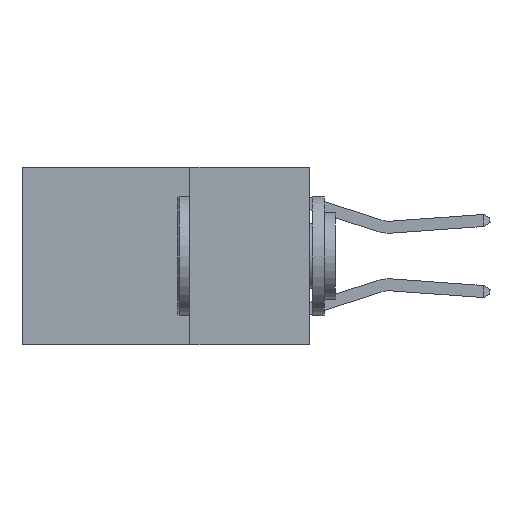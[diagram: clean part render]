
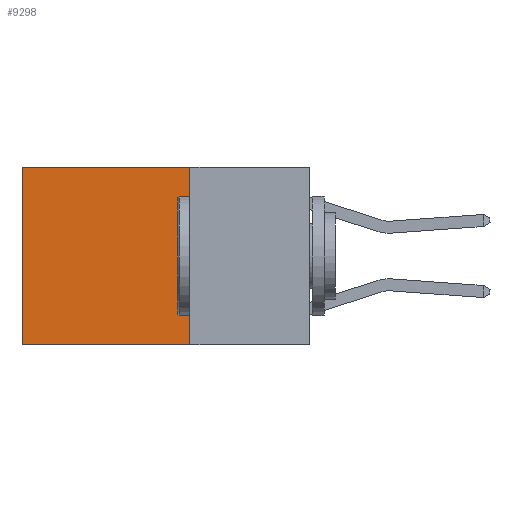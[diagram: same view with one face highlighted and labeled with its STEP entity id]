
A CAD part, left-side view. The second image highlights one B-rep face of the part: STEP entity #9298.
In plain terms, the highlighted planar face has unit normal (-1, 0, 0).
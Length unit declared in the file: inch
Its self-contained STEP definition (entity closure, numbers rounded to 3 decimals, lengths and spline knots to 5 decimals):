
#360 = CARTESIAN_POINT ( 'NONE',  ( 0.2625, 0.6, 0. ) ) ;
#2019 = ORIENTED_EDGE ( 'NONE', *, *, #15104, .T. ) ;
#3660 = EDGE_CURVE ( 'NONE', #13082, #6608, #14010, .T. ) ;
#4370 = CARTESIAN_POINT ( 'NONE',  ( 0.2625, 0.25, 0. ) ) ;
#5119 = CARTESIAN_POINT ( 'NONE',  ( 0.2625, 0.6, -0.37 ) ) ;
#5127 = DIRECTION ( 'NONE',  ( 0., 0., -1. ) ) ;
#5336 = VERTEX_POINT ( 'NONE', #360 ) ;
#5472 = EDGE_LOOP ( 'NONE', ( #15968, #21824, #13551, #2019 ) ) ;
#6608 = VERTEX_POINT ( 'NONE', #10085 ) ;
#7561 = CARTESIAN_POINT ( 'NONE',  ( 0.2625, 0.25, -0.37 ) ) ;
#7614 = EDGE_CURVE ( 'NONE', #6608, #17154, #20741, .T. ) ;
#9298 = ADVANCED_FACE ( 'NONE', ( #10443 ), #21840, .F. ) ;
#9308 = EDGE_CURVE ( 'NONE', #5336, #17154, #11889, .T. ) ;
#9544 = VECTOR ( 'NONE', #13009, 39.37008 ) ;
#9909 = AXIS2_PLACEMENT_3D ( 'NONE', #20397, #15441, #5127 ) ;
#10085 = CARTESIAN_POINT ( 'NONE',  ( 0.2625, 0.25, -0.37 ) ) ;
#10443 = FACE_OUTER_BOUND ( 'NONE', #5472, .T. ) ;
#11699 = VECTOR ( 'NONE', #19201, 39.37008 ) ;
#11889 = LINE ( 'NONE', #15221, #15578 ) ;
#12363 = CARTESIAN_POINT ( 'NONE',  ( 0.2625, 0.25, 0. ) ) ;
#12800 = LINE ( 'NONE', #12363, #11699 ) ;
#13009 = DIRECTION ( 'NONE',  ( 0., 0., -1. ) ) ;
#13082 = VERTEX_POINT ( 'NONE', #19485 ) ;
#13551 = ORIENTED_EDGE ( 'NONE', *, *, #3660, .F. ) ;
#14010 = LINE ( 'NONE', #4370, #9544 ) ;
#15104 = EDGE_CURVE ( 'NONE', #13082, #5336, #12800, .T. ) ;
#15221 = CARTESIAN_POINT ( 'NONE',  ( 0.2625, 0.6, 0. ) ) ;
#15441 = DIRECTION ( 'NONE',  ( 1., 0., 0. ) ) ;
#15578 = VECTOR ( 'NONE', #16981, 39.37008 ) ;
#15674 = DIRECTION ( 'NONE',  ( 0., 1., 0. ) ) ;
#15968 = ORIENTED_EDGE ( 'NONE', *, *, #9308, .T. ) ;
#16981 = DIRECTION ( 'NONE',  ( 0., 0., -1. ) ) ;
#17154 = VERTEX_POINT ( 'NONE', #5119 ) ;
#19201 = DIRECTION ( 'NONE',  ( 0., 1., 0. ) ) ;
#19485 = CARTESIAN_POINT ( 'NONE',  ( 0.2625, 0.25, 0. ) ) ;
#20397 = CARTESIAN_POINT ( 'NONE',  ( 0.2625, 0.25, 0. ) ) ;
#20741 = LINE ( 'NONE', #7561, #21820 ) ;
#21820 = VECTOR ( 'NONE', #15674, 39.37008 ) ;
#21824 = ORIENTED_EDGE ( 'NONE', *, *, #7614, .F. ) ;
#21840 = PLANE ( 'NONE',  #9909 ) ;
